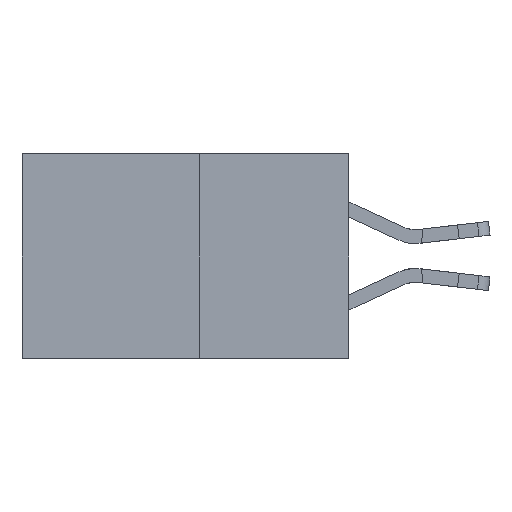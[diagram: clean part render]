
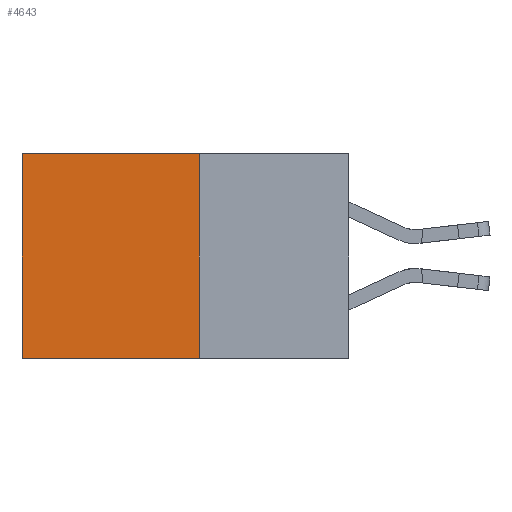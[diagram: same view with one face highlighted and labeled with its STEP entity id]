
A CAD part, left-side view. The second image highlights one B-rep face of the part: STEP entity #4643.
In plain terms, the highlighted planar face has unit normal (-1, 0, 0).
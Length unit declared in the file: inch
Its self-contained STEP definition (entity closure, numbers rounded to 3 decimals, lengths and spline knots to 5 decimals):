
#780 = VERTEX_POINT ( 'NONE', #16831 ) ;
#1256 = CARTESIAN_POINT ( 'NONE',  ( 0.277, 0.27, -0.37 ) ) ;
#1273 = ORIENTED_EDGE ( 'NONE', *, *, #20458, .F. ) ;
#3632 = VECTOR ( 'NONE', #10050, 39.37008 ) ;
#4193 = EDGE_CURVE ( 'NONE', #18868, #780, #4213, .T. ) ;
#4213 = LINE ( 'NONE', #9968, #3632 ) ;
#4417 = ORIENTED_EDGE ( 'NONE', *, *, #22114, .F. ) ;
#4475 = DIRECTION ( 'NONE',  ( 0., 0., -1. ) ) ;
#4528 = DIRECTION ( 'NONE',  ( 1., 0., 0. ) ) ;
#4557 = CARTESIAN_POINT ( 'NONE',  ( 0.277, 0.27, -0.37 ) ) ;
#4611 = PLANE ( 'NONE',  #20410 ) ;
#4643 = ADVANCED_FACE ( 'NONE', ( #23045 ), #4611, .F. ) ;
#4896 = VERTEX_POINT ( 'NONE', #1256 ) ;
#7725 = VECTOR ( 'NONE', #8561, 39.37008 ) ;
#7747 = EDGE_LOOP ( 'NONE', ( #11967, #1273, #4417, #8041 ) ) ;
#8041 = ORIENTED_EDGE ( 'NONE', *, *, #21456, .T. ) ;
#8503 = DIRECTION ( 'NONE',  ( 0., 1., 0. ) ) ;
#8530 = DIRECTION ( 'NONE',  ( 0., 0., -1. ) ) ;
#8561 = DIRECTION ( 'NONE',  ( 0., 1., 0. ) ) ;
#9769 = LINE ( 'NONE', #17999, #24226 ) ;
#9968 = CARTESIAN_POINT ( 'NONE',  ( 0.277, 0.59, -0.37 ) ) ;
#10050 = DIRECTION ( 'NONE',  ( 0., 0., -1. ) ) ;
#11586 = VERTEX_POINT ( 'NONE', #21392 ) ;
#11967 = ORIENTED_EDGE ( 'NONE', *, *, #4193, .T. ) ;
#12940 = VECTOR ( 'NONE', #8530, 39.37008 ) ;
#16831 = CARTESIAN_POINT ( 'NONE',  ( 0.277, 0.59, -0.37 ) ) ;
#17973 = CARTESIAN_POINT ( 'NONE',  ( 0.277, 0.27, 0. ) ) ;
#17999 = CARTESIAN_POINT ( 'NONE',  ( 0.277, 0.27, -0.37 ) ) ;
#18868 = VERTEX_POINT ( 'NONE', #21316 ) ;
#19873 = CARTESIAN_POINT ( 'NONE',  ( 0.277, 0.27, -0.37 ) ) ;
#20410 = AXIS2_PLACEMENT_3D ( 'NONE', #4557, #4528, #4475 ) ;
#20458 = EDGE_CURVE ( 'NONE', #4896, #780, #9769, .T. ) ;
#21316 = CARTESIAN_POINT ( 'NONE',  ( 0.277, 0.59, 0. ) ) ;
#21392 = CARTESIAN_POINT ( 'NONE',  ( 0.277, 0.27, 0. ) ) ;
#21456 = EDGE_CURVE ( 'NONE', #11586, #18868, #22757, .T. ) ;
#22114 = EDGE_CURVE ( 'NONE', #11586, #4896, #22439, .T. ) ;
#22439 = LINE ( 'NONE', #19873, #12940 ) ;
#22757 = LINE ( 'NONE', #17973, #7725 ) ;
#23045 = FACE_OUTER_BOUND ( 'NONE', #7747, .T. ) ;
#24226 = VECTOR ( 'NONE', #8503, 39.37008 ) ;
